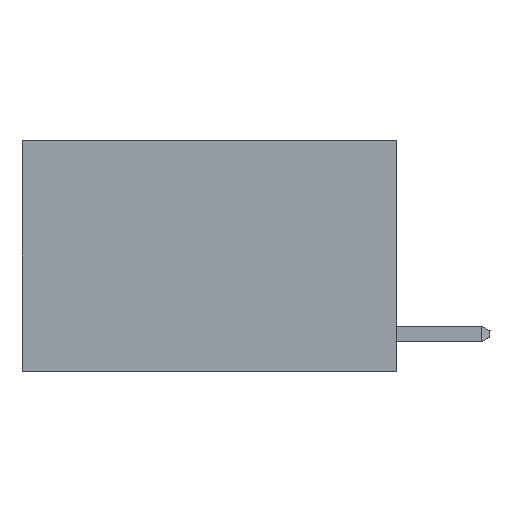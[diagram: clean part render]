
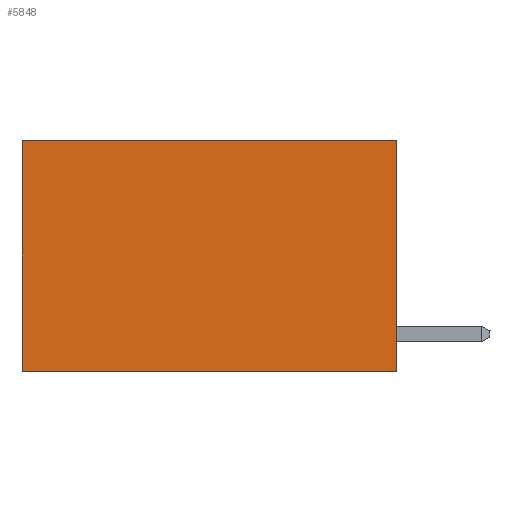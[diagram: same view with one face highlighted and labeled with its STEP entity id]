
A CAD part, left-side view. The second image highlights one B-rep face of the part: STEP entity #5848.
In plain terms, the highlighted planar face has unit normal (-1, 0, 0).
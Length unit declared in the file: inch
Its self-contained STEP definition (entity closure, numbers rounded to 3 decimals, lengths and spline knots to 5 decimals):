
#676 = ORIENTED_EDGE ( 'NONE', *, *, #10939, .F. ) ;
#716 = CARTESIAN_POINT ( 'NONE',  ( 0.2625, 0.6, 0. ) ) ;
#1418 = VECTOR ( 'NONE', #12129, 39.37008 ) ;
#1764 = DIRECTION ( 'NONE',  ( 0., 1., 0. ) ) ;
#1877 = VERTEX_POINT ( 'NONE', #8928 ) ;
#2127 = DIRECTION ( 'NONE',  ( 1., 0., 0. ) ) ;
#2544 = AXIS2_PLACEMENT_3D ( 'NONE', #6355, #2127, #9433 ) ;
#2698 = VERTEX_POINT ( 'NONE', #9448 ) ;
#3307 = LINE ( 'NONE', #7350, #6179 ) ;
#3390 = ORIENTED_EDGE ( 'NONE', *, *, #6176, .F. ) ;
#3556 = VERTEX_POINT ( 'NONE', #5949 ) ;
#4822 = CARTESIAN_POINT ( 'NONE',  ( 0.2625, 0., -0.37 ) ) ;
#5148 = DIRECTION ( 'NONE',  ( 0., 0., -1. ) ) ;
#5848 = ADVANCED_FACE ( 'NONE', ( #9876 ), #9392, .F. ) ;
#5949 = CARTESIAN_POINT ( 'NONE',  ( 0.2625, 0.6, -0.37 ) ) ;
#5983 = VERTEX_POINT ( 'NONE', #12727 ) ;
#6176 = EDGE_CURVE ( 'NONE', #1877, #5983, #3307, .T. ) ;
#6179 = VECTOR ( 'NONE', #5148, 39.37008 ) ;
#6355 = CARTESIAN_POINT ( 'NONE',  ( 0.2625, 0., 0. ) ) ;
#6501 = VECTOR ( 'NONE', #1764, 39.37008 ) ;
#6720 = EDGE_LOOP ( 'NONE', ( #11367, #676, #3390, #11670 ) ) ;
#6839 = LINE ( 'NONE', #4822, #6501 ) ;
#7331 = VECTOR ( 'NONE', #12065, 39.37008 ) ;
#7350 = CARTESIAN_POINT ( 'NONE',  ( 0.2625, 0., 0. ) ) ;
#8759 = EDGE_CURVE ( 'NONE', #1877, #2698, #9730, .T. ) ;
#8928 = CARTESIAN_POINT ( 'NONE',  ( 0.2625, 0., 0. ) ) ;
#9392 = PLANE ( 'NONE',  #2544 ) ;
#9433 = DIRECTION ( 'NONE',  ( 0., 0., -1. ) ) ;
#9448 = CARTESIAN_POINT ( 'NONE',  ( 0.2625, 0.6, 0. ) ) ;
#9730 = LINE ( 'NONE', #11145, #1418 ) ;
#9876 = FACE_OUTER_BOUND ( 'NONE', #6720, .T. ) ;
#9998 = LINE ( 'NONE', #716, #7331 ) ;
#10939 = EDGE_CURVE ( 'NONE', #5983, #3556, #6839, .T. ) ;
#11145 = CARTESIAN_POINT ( 'NONE',  ( 0.2625, 0., 0. ) ) ;
#11367 = ORIENTED_EDGE ( 'NONE', *, *, #11780, .T. ) ;
#11670 = ORIENTED_EDGE ( 'NONE', *, *, #8759, .T. ) ;
#11780 = EDGE_CURVE ( 'NONE', #2698, #3556, #9998, .T. ) ;
#12065 = DIRECTION ( 'NONE',  ( 0., 0., -1. ) ) ;
#12129 = DIRECTION ( 'NONE',  ( 0., 1., 0. ) ) ;
#12727 = CARTESIAN_POINT ( 'NONE',  ( 0.2625, 0., -0.37 ) ) ;
